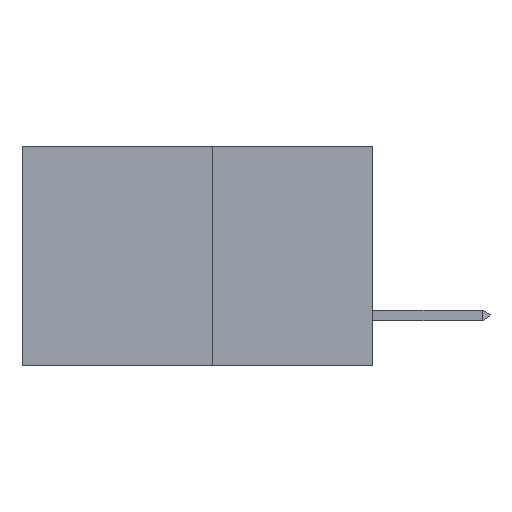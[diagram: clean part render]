
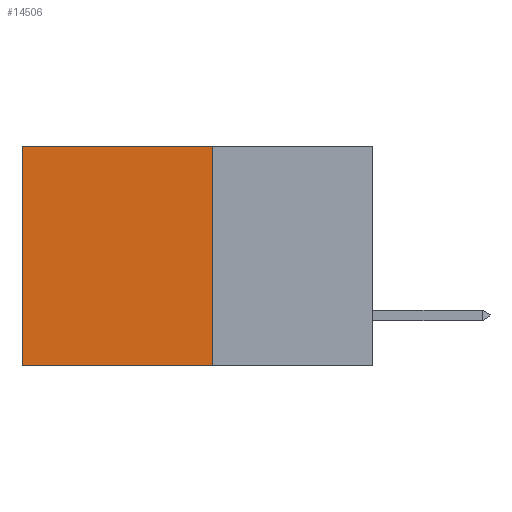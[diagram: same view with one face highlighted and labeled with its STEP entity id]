
A CAD part, left-side view. The second image highlights one B-rep face of the part: STEP entity #14506.
In plain terms, the highlighted planar face has unit normal (-1, 0, 0).
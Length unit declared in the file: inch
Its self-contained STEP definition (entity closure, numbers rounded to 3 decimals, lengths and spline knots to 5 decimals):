
#301 = VERTEX_POINT ( 'NONE', #6711 ) ;
#1260 = ORIENTED_EDGE ( 'NONE', *, *, #1906, .F. ) ;
#1759 = EDGE_CURVE ( 'NONE', #9573, #14496, #11342, .T. ) ;
#1795 = CARTESIAN_POINT ( 'NONE',  ( 0.277, 0.59, -0.37 ) ) ;
#1848 = CARTESIAN_POINT ( 'NONE',  ( 0.277, 0.27, 0. ) ) ;
#1906 = EDGE_CURVE ( 'NONE', #3327, #301, #5584, .T. ) ;
#2390 = DIRECTION ( 'NONE',  ( 0., 1., 0. ) ) ;
#2959 = CARTESIAN_POINT ( 'NONE',  ( 0.277, 0.27, 0. ) ) ;
#3327 = VERTEX_POINT ( 'NONE', #11974 ) ;
#3445 = DIRECTION ( 'NONE',  ( 0., 0., -1. ) ) ;
#3550 = ORIENTED_EDGE ( 'NONE', *, *, #1759, .T. ) ;
#4568 = CARTESIAN_POINT ( 'NONE',  ( 0.277, 0.27, -0.37 ) ) ;
#5584 = LINE ( 'NONE', #8052, #14059 ) ;
#5930 = PLANE ( 'NONE',  #14664 ) ;
#6255 = DIRECTION ( 'NONE',  ( 0., 0., -1. ) ) ;
#6312 = LINE ( 'NONE', #4568, #14761 ) ;
#6711 = CARTESIAN_POINT ( 'NONE',  ( 0.277, 0.59, -0.37 ) ) ;
#6763 = VECTOR ( 'NONE', #2390, 39.37008 ) ;
#7601 = CARTESIAN_POINT ( 'NONE',  ( 0.277, 0.59, 0. ) ) ;
#8052 = CARTESIAN_POINT ( 'NONE',  ( 0.277, 0.27, -0.37 ) ) ;
#9385 = DIRECTION ( 'NONE',  ( 1., 0., 0. ) ) ;
#9573 = VERTEX_POINT ( 'NONE', #2959 ) ;
#10415 = FACE_OUTER_BOUND ( 'NONE', #19667, .T. ) ;
#11342 = LINE ( 'NONE', #1848, #6763 ) ;
#11974 = CARTESIAN_POINT ( 'NONE',  ( 0.277, 0.27, -0.37 ) ) ;
#13031 = LINE ( 'NONE', #1795, #21291 ) ;
#14059 = VECTOR ( 'NONE', #18050, 39.37008 ) ;
#14496 = VERTEX_POINT ( 'NONE', #7601 ) ;
#14506 = ADVANCED_FACE ( 'NONE', ( #10415 ), #5930, .F. ) ;
#14664 = AXIS2_PLACEMENT_3D ( 'NONE', #19363, #9385, #21001 ) ;
#14761 = VECTOR ( 'NONE', #6255, 39.37008 ) ;
#16460 = EDGE_CURVE ( 'NONE', #9573, #3327, #6312, .T. ) ;
#17863 = ORIENTED_EDGE ( 'NONE', *, *, #16460, .F. ) ;
#18050 = DIRECTION ( 'NONE',  ( 0., 1., 0. ) ) ;
#19363 = CARTESIAN_POINT ( 'NONE',  ( 0.277, 0.27, -0.37 ) ) ;
#19667 = EDGE_LOOP ( 'NONE', ( #19888, #1260, #17863, #3550 ) ) ;
#19888 = ORIENTED_EDGE ( 'NONE', *, *, #20470, .T. ) ;
#20470 = EDGE_CURVE ( 'NONE', #14496, #301, #13031, .T. ) ;
#21001 = DIRECTION ( 'NONE',  ( 0., 0., -1. ) ) ;
#21291 = VECTOR ( 'NONE', #3445, 39.37008 ) ;
